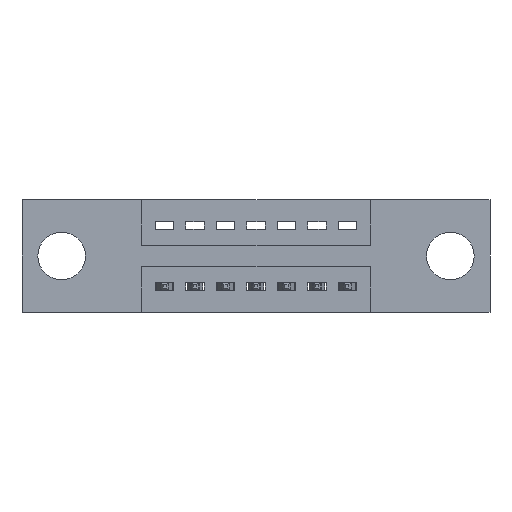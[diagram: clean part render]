
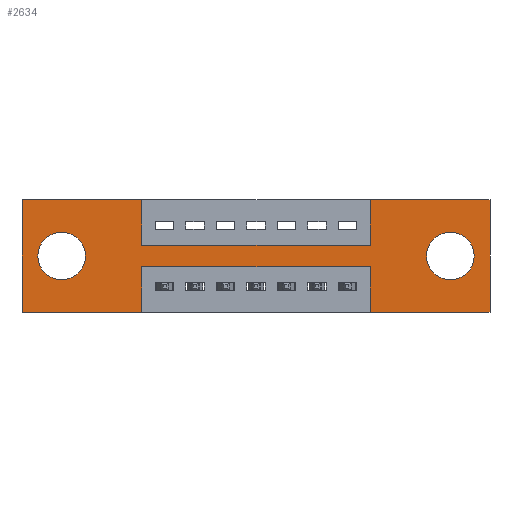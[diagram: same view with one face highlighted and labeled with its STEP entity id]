
A CAD part, front view. The second image highlights one B-rep face of the part: STEP entity #2634.
In plain terms, the highlighted planar face has unit normal (0, -1, 0).
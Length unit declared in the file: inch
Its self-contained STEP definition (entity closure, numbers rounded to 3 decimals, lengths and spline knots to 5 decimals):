
#10 = DIRECTION ( 'NONE',  ( 1., 0., 0. ) ) ;
#39 = EDGE_CURVE ( 'NONE', #3576, #9207, #751, .T. ) ;
#122 = CARTESIAN_POINT ( 'NONE',  ( 0.3925, 0., -0.37 ) ) ;
#292 = VECTOR ( 'NONE', #1577, 39.37008 ) ;
#301 = CARTESIAN_POINT ( 'NONE',  ( 0.13, 0., -0.185 ) ) ;
#355 = EDGE_CURVE ( 'NONE', #6177, #1103, #7630, .T. ) ;
#456 = ORIENTED_EDGE ( 'NONE', *, *, #3394, .F. ) ;
#457 = DIRECTION ( 'NONE',  ( 0., 0., -1. ) ) ;
#471 = EDGE_CURVE ( 'NONE', #9207, #3576, #1450, .T. ) ;
#488 = CARTESIAN_POINT ( 'NONE',  ( 1.1425, 0., -0.37 ) ) ;
#511 = DIRECTION ( 'NONE',  ( -1., 0., 0. ) ) ;
#564 = CIRCLE ( 'NONE', #7349, 0.078 ) ;
#588 = PLANE ( 'NONE',  #4005 ) ;
#617 = EDGE_CURVE ( 'NONE', #1096, #5908, #7853, .T. ) ;
#695 = EDGE_LOOP ( 'NONE', ( #1072, #3078 ) ) ;
#751 = CIRCLE ( 'NONE', #3499, 0.078 ) ;
#755 = CARTESIAN_POINT ( 'NONE',  ( 0.3925, 0., -0.37 ) ) ;
#854 = DIRECTION ( 'NONE',  ( 0., 0., -1. ) ) ;
#1072 = ORIENTED_EDGE ( 'NONE', *, *, #471, .T. ) ;
#1096 = VERTEX_POINT ( 'NONE', #6134 ) ;
#1103 = VERTEX_POINT ( 'NONE', #2271 ) ;
#1220 = ORIENTED_EDGE ( 'NONE', *, *, #1371, .F. ) ;
#1371 = EDGE_CURVE ( 'NONE', #3626, #3888, #8096, .T. ) ;
#1450 = CIRCLE ( 'NONE', #2270, 0.078 ) ;
#1577 = DIRECTION ( 'NONE',  ( 0., 0., -1. ) ) ;
#1600 = EDGE_CURVE ( 'NONE', #1103, #5906, #10013, .T. ) ;
#1644 = ORIENTED_EDGE ( 'NONE', *, *, #1600, .F. ) ;
#1725 = DIRECTION ( 'NONE',  ( 0., 1., 0. ) ) ;
#1745 = EDGE_CURVE ( 'NONE', #3240, #8780, #3794, .T. ) ;
#1765 = CARTESIAN_POINT ( 'NONE',  ( 1.405, 0., -0.185 ) ) ;
#1864 = CARTESIAN_POINT ( 'NONE',  ( 1.1425, 0., -0.22 ) ) ;
#1865 = LINE ( 'NONE', #9135, #9852 ) ;
#1873 = DIRECTION ( 'NONE',  ( 0., 0., -1. ) ) ;
#2029 = CARTESIAN_POINT ( 'NONE',  ( 1.1425, 0., 0. ) ) ;
#2030 = CARTESIAN_POINT ( 'NONE',  ( 0., 0., -0.37 ) ) ;
#2180 = ORIENTED_EDGE ( 'NONE', *, *, #5766, .F. ) ;
#2270 = AXIS2_PLACEMENT_3D ( 'NONE', #2880, #6179, #8295 ) ;
#2271 = CARTESIAN_POINT ( 'NONE',  ( 1.535, 0., -0.37 ) ) ;
#2323 = VERTEX_POINT ( 'NONE', #3940 ) ;
#2634 = ADVANCED_FACE ( 'NONE', ( #5753, #8317, #5369 ), #588, .T. ) ;
#2880 = CARTESIAN_POINT ( 'NONE',  ( 0.13, 0., -0.185 ) ) ;
#3078 = ORIENTED_EDGE ( 'NONE', *, *, #39, .T. ) ;
#3240 = VERTEX_POINT ( 'NONE', #6695 ) ;
#3394 = EDGE_CURVE ( 'NONE', #9673, #2323, #5472, .T. ) ;
#3499 = AXIS2_PLACEMENT_3D ( 'NONE', #301, #1725, #5822 ) ;
#3576 = VERTEX_POINT ( 'NONE', #6878 ) ;
#3589 = EDGE_CURVE ( 'NONE', #3888, #8959, #9359, .T. ) ;
#3626 = VERTEX_POINT ( 'NONE', #1864 ) ;
#3766 = EDGE_CURVE ( 'NONE', #8959, #9673, #4860, .T. ) ;
#3794 = CIRCLE ( 'NONE', #7031, 0.078 ) ;
#3847 = CARTESIAN_POINT ( 'NONE',  ( 0., 0., -0.37 ) ) ;
#3888 = VERTEX_POINT ( 'NONE', #6049 ) ;
#3923 = VECTOR ( 'NONE', #5827, 39.37008 ) ;
#3940 = CARTESIAN_POINT ( 'NONE',  ( 0., 0., 0. ) ) ;
#3957 = EDGE_CURVE ( 'NONE', #2323, #4016, #1865, .T. ) ;
#4005 = AXIS2_PLACEMENT_3D ( 'NONE', #2030, #5061, #457 ) ;
#4016 = VERTEX_POINT ( 'NONE', #5173 ) ;
#4135 = VECTOR ( 'NONE', #854, 39.37008 ) ;
#4141 = VERTEX_POINT ( 'NONE', #5551 ) ;
#4389 = LINE ( 'NONE', #4545, #4732 ) ;
#4441 = CARTESIAN_POINT ( 'NONE',  ( 0., 0., -0.37 ) ) ;
#4545 = CARTESIAN_POINT ( 'NONE',  ( 1.1425, 0., -0.37 ) ) ;
#4732 = VECTOR ( 'NONE', #9991, 39.37008 ) ;
#4857 = EDGE_LOOP ( 'NONE', ( #7024, #1220, #6003, #1644, #6140, #5159, #5820, #2180, #6334, #7320, #456, #8866 ) ) ;
#4858 = LINE ( 'NONE', #6225, #292 ) ;
#4860 = LINE ( 'NONE', #9800, #8506 ) ;
#4932 = CARTESIAN_POINT ( 'NONE',  ( 1.405, 0., -0.185 ) ) ;
#5061 = DIRECTION ( 'NONE',  ( 0., -1., 0. ) ) ;
#5159 = ORIENTED_EDGE ( 'NONE', *, *, #7453, .F. ) ;
#5173 = CARTESIAN_POINT ( 'NONE',  ( 0.3925, 0., 0. ) ) ;
#5369 = FACE_OUTER_BOUND ( 'NONE', #4857, .T. ) ;
#5384 = VECTOR ( 'NONE', #9335, 39.37008 ) ;
#5416 = CARTESIAN_POINT ( 'NONE',  ( 0.13, 0., -0.107 ) ) ;
#5472 = LINE ( 'NONE', #5947, #7574 ) ;
#5551 = CARTESIAN_POINT ( 'NONE',  ( 0.3925, 0., -0.15 ) ) ;
#5753 = FACE_BOUND ( 'NONE', #6057, .T. ) ;
#5766 = EDGE_CURVE ( 'NONE', #4141, #1096, #8710, .T. ) ;
#5802 = DIRECTION ( 'NONE',  ( 1., 0., 0. ) ) ;
#5820 = ORIENTED_EDGE ( 'NONE', *, *, #617, .F. ) ;
#5822 = DIRECTION ( 'NONE',  ( 0., 0., 1. ) ) ;
#5827 = DIRECTION ( 'NONE',  ( -1., 0., 0. ) ) ;
#5846 = CARTESIAN_POINT ( 'NONE',  ( 1.535, 0., 0. ) ) ;
#5894 = CARTESIAN_POINT ( 'NONE',  ( 0.3925, 0., -0.15 ) ) ;
#5906 = VERTEX_POINT ( 'NONE', #488 ) ;
#5908 = VERTEX_POINT ( 'NONE', #2029 ) ;
#5916 = VECTOR ( 'NONE', #10, 39.37008 ) ;
#5947 = CARTESIAN_POINT ( 'NONE',  ( 0., 0., 0. ) ) ;
#6003 = ORIENTED_EDGE ( 'NONE', *, *, #8117, .F. ) ;
#6049 = CARTESIAN_POINT ( 'NONE',  ( 0.3925, 0., -0.22 ) ) ;
#6057 = EDGE_LOOP ( 'NONE', ( #9482, #6097 ) ) ;
#6097 = ORIENTED_EDGE ( 'NONE', *, *, #7706, .T. ) ;
#6134 = CARTESIAN_POINT ( 'NONE',  ( 1.1425, 0., -0.15 ) ) ;
#6140 = ORIENTED_EDGE ( 'NONE', *, *, #355, .F. ) ;
#6177 = VERTEX_POINT ( 'NONE', #9573 ) ;
#6179 = DIRECTION ( 'NONE',  ( 0., 1., 0. ) ) ;
#6225 = CARTESIAN_POINT ( 'NONE',  ( 0.3925, 0., 0. ) ) ;
#6334 = ORIENTED_EDGE ( 'NONE', *, *, #8829, .F. ) ;
#6633 = VECTOR ( 'NONE', #5802, 39.37008 ) ;
#6695 = CARTESIAN_POINT ( 'NONE',  ( 1.405, 0., -0.107 ) ) ;
#6878 = CARTESIAN_POINT ( 'NONE',  ( 0.13, 0., -0.263 ) ) ;
#6901 = VECTOR ( 'NONE', #7725, 39.37008 ) ;
#7024 = ORIENTED_EDGE ( 'NONE', *, *, #3589, .F. ) ;
#7031 = AXIS2_PLACEMENT_3D ( 'NONE', #1765, #7262, #7190 ) ;
#7190 = DIRECTION ( 'NONE',  ( 0., 0., -1. ) ) ;
#7262 = DIRECTION ( 'NONE',  ( 0., 1., 0. ) ) ;
#7320 = ORIENTED_EDGE ( 'NONE', *, *, #3957, .F. ) ;
#7349 = AXIS2_PLACEMENT_3D ( 'NONE', #4932, #8025, #1873 ) ;
#7453 = EDGE_CURVE ( 'NONE', #5908, #6177, #9507, .T. ) ;
#7574 = VECTOR ( 'NONE', #8338, 39.37008 ) ;
#7630 = LINE ( 'NONE', #5846, #8465 ) ;
#7706 = EDGE_CURVE ( 'NONE', #8780, #3240, #564, .T. ) ;
#7725 = DIRECTION ( 'NONE',  ( 0., 0., 1. ) ) ;
#7760 = CARTESIAN_POINT ( 'NONE',  ( 1.1425, 0., 0. ) ) ;
#7853 = LINE ( 'NONE', #7760, #6901 ) ;
#8025 = DIRECTION ( 'NONE',  ( 0., 1., 0. ) ) ;
#8096 = LINE ( 'NONE', #8203, #3923 ) ;
#8117 = EDGE_CURVE ( 'NONE', #5906, #3626, #4389, .T. ) ;
#8132 = DIRECTION ( 'NONE',  ( 0., 0., -1. ) ) ;
#8203 = CARTESIAN_POINT ( 'NONE',  ( 0.3925, 0., -0.22 ) ) ;
#8295 = DIRECTION ( 'NONE',  ( 0., 0., 1. ) ) ;
#8317 = FACE_BOUND ( 'NONE', #695, .T. ) ;
#8338 = DIRECTION ( 'NONE',  ( 0., 0., 1. ) ) ;
#8465 = VECTOR ( 'NONE', #8132, 39.37008 ) ;
#8506 = VECTOR ( 'NONE', #511, 39.37008 ) ;
#8710 = LINE ( 'NONE', #5894, #5916 ) ;
#8780 = VERTEX_POINT ( 'NONE', #9864 ) ;
#8829 = EDGE_CURVE ( 'NONE', #4016, #4141, #4858, .T. ) ;
#8866 = ORIENTED_EDGE ( 'NONE', *, *, #3766, .F. ) ;
#8959 = VERTEX_POINT ( 'NONE', #122 ) ;
#9135 = CARTESIAN_POINT ( 'NONE',  ( 0., 0., 0. ) ) ;
#9170 = DIRECTION ( 'NONE',  ( 1., 0., 0. ) ) ;
#9207 = VERTEX_POINT ( 'NONE', #5416 ) ;
#9335 = DIRECTION ( 'NONE',  ( -1., 0., 0. ) ) ;
#9359 = LINE ( 'NONE', #755, #4135 ) ;
#9482 = ORIENTED_EDGE ( 'NONE', *, *, #1745, .T. ) ;
#9507 = LINE ( 'NONE', #9668, #6633 ) ;
#9573 = CARTESIAN_POINT ( 'NONE',  ( 1.535, 0., 0. ) ) ;
#9668 = CARTESIAN_POINT ( 'NONE',  ( 0., 0., 0. ) ) ;
#9673 = VERTEX_POINT ( 'NONE', #4441 ) ;
#9800 = CARTESIAN_POINT ( 'NONE',  ( 0., 0., -0.37 ) ) ;
#9852 = VECTOR ( 'NONE', #9170, 39.37008 ) ;
#9864 = CARTESIAN_POINT ( 'NONE',  ( 1.405, 0., -0.263 ) ) ;
#9991 = DIRECTION ( 'NONE',  ( 0., 0., 1. ) ) ;
#10013 = LINE ( 'NONE', #3847, #5384 ) ;
